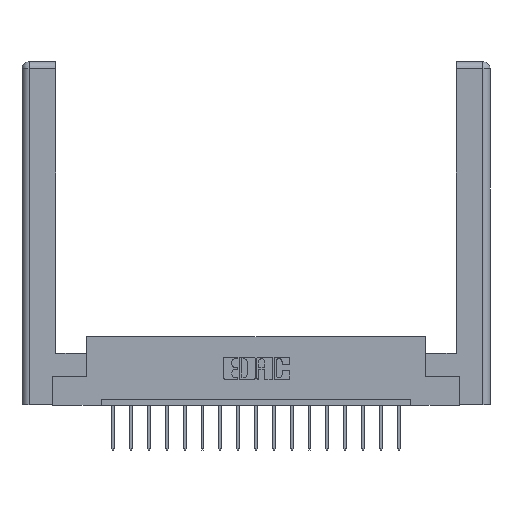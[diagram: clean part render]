
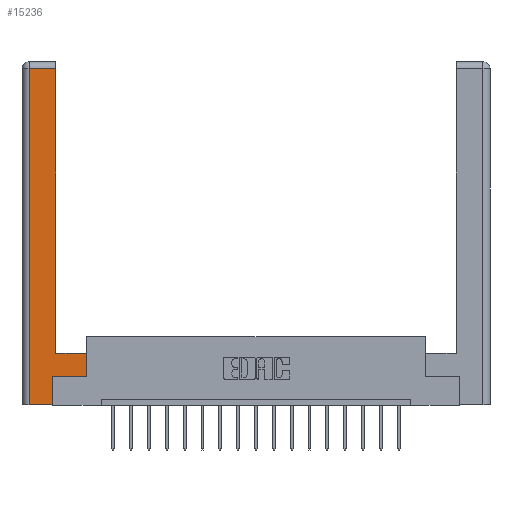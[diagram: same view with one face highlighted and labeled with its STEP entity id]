
A CAD part, top view. The second image highlights one B-rep face of the part: STEP entity #15236.
In plain terms, the highlighted planar face has unit normal (0, 0, 1).
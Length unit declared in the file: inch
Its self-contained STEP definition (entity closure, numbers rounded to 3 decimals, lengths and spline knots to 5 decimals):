
#61 = FACE_OUTER_BOUND ( 'NONE', #9626, .T. ) ;
#315 = CARTESIAN_POINT ( 'NONE',  ( 0.295, 3., 0. ) ) ;
#1255 = VERTEX_POINT ( 'NONE', #15577 ) ;
#1418 = EDGE_CURVE ( 'NONE', #18367, #1255, #8185, .T. ) ;
#1531 = ORIENTED_EDGE ( 'NONE', *, *, #14951, .T. ) ;
#1547 = DIRECTION ( 'NONE',  ( -1., 0., 0. ) ) ;
#1697 = CARTESIAN_POINT ( 'NONE',  ( 0.0615, 2.94, 0. ) ) ;
#2017 = EDGE_CURVE ( 'NONE', #10162, #15838, #16313, .T. ) ;
#2306 = DIRECTION ( 'NONE',  ( -1., 0., 0. ) ) ;
#2339 = VERTEX_POINT ( 'NONE', #11478 ) ;
#2461 = VECTOR ( 'NONE', #14394, 39.37008 ) ;
#2586 = VECTOR ( 'NONE', #10321, 39.37008 ) ;
#2831 = CARTESIAN_POINT ( 'NONE',  ( 0.565, 0.245, 0. ) ) ;
#2869 = VECTOR ( 'NONE', #7832, 39.37008 ) ;
#3061 = ORIENTED_EDGE ( 'NONE', *, *, #2017, .T. ) ;
#3346 = VERTEX_POINT ( 'NONE', #12888 ) ;
#3494 = CARTESIAN_POINT ( 'NONE',  ( 0.265, 0.245, 0. ) ) ;
#3627 = CARTESIAN_POINT ( 'NONE',  ( 0.295, 0.45, 0. ) ) ;
#3706 = DIRECTION ( 'NONE',  ( -1., 0., 0. ) ) ;
#3905 = VERTEX_POINT ( 'NONE', #8343 ) ;
#4062 = DIRECTION ( 'NONE',  ( 0., 1., 0. ) ) ;
#4321 = PLANE ( 'NONE',  #9006 ) ;
#4567 = CARTESIAN_POINT ( 'NONE',  ( 0.565, 0.45, 0. ) ) ;
#4713 = VECTOR ( 'NONE', #2306, 39.37008 ) ;
#5434 = EDGE_CURVE ( 'NONE', #3346, #2339, #14454, .T. ) ;
#6029 = ORIENTED_EDGE ( 'NONE', *, *, #11864, .T. ) ;
#6275 = VECTOR ( 'NONE', #14961, 39.37008 ) ;
#6326 = CARTESIAN_POINT ( 'NONE',  ( 0.265, 0.245, 0. ) ) ;
#7230 = EDGE_CURVE ( 'NONE', #11415, #3346, #8565, .T. ) ;
#7832 = DIRECTION ( 'NONE',  ( 0., -1., 0. ) ) ;
#7937 = ORIENTED_EDGE ( 'NONE', *, *, #7230, .T. ) ;
#8136 = LINE ( 'NONE', #1697, #8368 ) ;
#8185 = LINE ( 'NONE', #13193, #11772 ) ;
#8196 = ORIENTED_EDGE ( 'NONE', *, *, #5434, .T. ) ;
#8343 = CARTESIAN_POINT ( 'NONE',  ( 0.0615, 2.94, 0. ) ) ;
#8368 = VECTOR ( 'NONE', #3706, 39.37008 ) ;
#8423 = LINE ( 'NONE', #12637, #9308 ) ;
#8565 = LINE ( 'NONE', #3627, #4713 ) ;
#8954 = DIRECTION ( 'NONE',  ( 1., 0., 0. ) ) ;
#9006 = AXIS2_PLACEMENT_3D ( 'NONE', #14390, #10133, #1547 ) ;
#9308 = VECTOR ( 'NONE', #4062, 39.37008 ) ;
#9626 = EDGE_LOOP ( 'NONE', ( #8196, #1531, #14067, #12991, #16553, #3061, #6029, #7937 ) ) ;
#9680 = CARTESIAN_POINT ( 'NONE',  ( 0.0615, 0., 0. ) ) ;
#10133 = DIRECTION ( 'NONE',  ( 0., 0., -1. ) ) ;
#10162 = VERTEX_POINT ( 'NONE', #3494 ) ;
#10321 = DIRECTION ( 'NONE',  ( 0., 1., 0. ) ) ;
#10471 = CARTESIAN_POINT ( 'NONE',  ( 0.565, 0.245, 0. ) ) ;
#10632 = CARTESIAN_POINT ( 'NONE',  ( 0.0615, 0., 0. ) ) ;
#11415 = VERTEX_POINT ( 'NONE', #4567 ) ;
#11478 = CARTESIAN_POINT ( 'NONE',  ( 0.295, 2.94, 0. ) ) ;
#11772 = VECTOR ( 'NONE', #8954, 39.37008 ) ;
#11864 = EDGE_CURVE ( 'NONE', #15838, #11415, #8423, .T. ) ;
#12637 = CARTESIAN_POINT ( 'NONE',  ( 0.565, 0.45, 0. ) ) ;
#12888 = CARTESIAN_POINT ( 'NONE',  ( 0.295, 0.45, 0. ) ) ;
#12991 = ORIENTED_EDGE ( 'NONE', *, *, #1418, .T. ) ;
#13193 = CARTESIAN_POINT ( 'NONE',  ( 0.265, 0., 0. ) ) ;
#13820 = EDGE_CURVE ( 'NONE', #1255, #10162, #18168, .T. ) ;
#14067 = ORIENTED_EDGE ( 'NONE', *, *, #17933, .T. ) ;
#14390 = CARTESIAN_POINT ( 'NONE',  ( 0., 0., 0. ) ) ;
#14394 = DIRECTION ( 'NONE',  ( 1., 0., 0. ) ) ;
#14454 = LINE ( 'NONE', #315, #2586 ) ;
#14951 = EDGE_CURVE ( 'NONE', #2339, #3905, #8136, .T. ) ;
#14961 = DIRECTION ( 'NONE',  ( 0., 1., 0. ) ) ;
#15236 = ADVANCED_FACE ( 'NONE', ( #61 ), #4321, .F. ) ;
#15577 = CARTESIAN_POINT ( 'NONE',  ( 0.265, 0., 0. ) ) ;
#15838 = VERTEX_POINT ( 'NONE', #10471 ) ;
#16313 = LINE ( 'NONE', #2831, #2461 ) ;
#16520 = LINE ( 'NONE', #10632, #2869 ) ;
#16553 = ORIENTED_EDGE ( 'NONE', *, *, #13820, .T. ) ;
#17933 = EDGE_CURVE ( 'NONE', #3905, #18367, #16520, .T. ) ;
#18168 = LINE ( 'NONE', #6326, #6275 ) ;
#18367 = VERTEX_POINT ( 'NONE', #9680 ) ;
